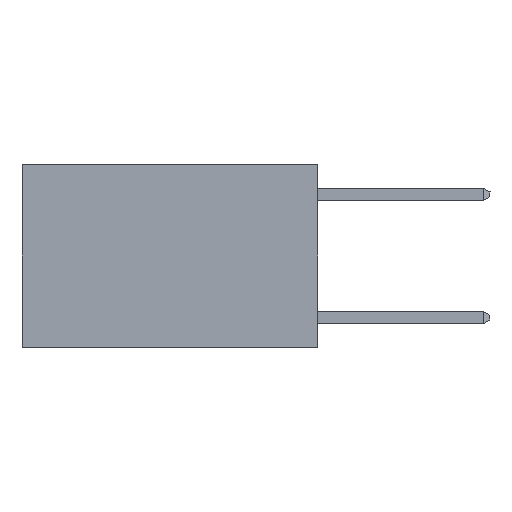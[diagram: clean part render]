
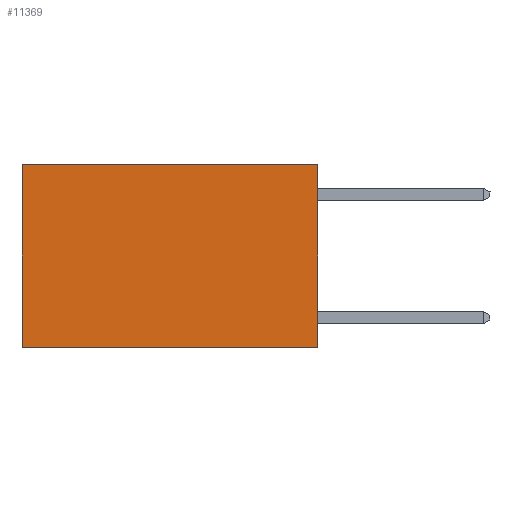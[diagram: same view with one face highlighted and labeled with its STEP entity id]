
A CAD part, left-side view. The second image highlights one B-rep face of the part: STEP entity #11369.
In plain terms, the highlighted planar face has unit normal (-1, 0, 0).
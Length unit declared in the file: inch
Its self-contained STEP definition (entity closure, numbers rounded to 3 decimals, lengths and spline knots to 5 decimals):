
#688 = CARTESIAN_POINT ( 'NONE',  ( 0.2625, 0., 0. ) ) ;
#1517 = PLANE ( 'NONE',  #5953 ) ;
#1941 = CARTESIAN_POINT ( 'NONE',  ( 0.2625, 0., 0. ) ) ;
#2280 = LINE ( 'NONE', #6878, #8079 ) ;
#2660 = DIRECTION ( 'NONE',  ( 0., 0., -1. ) ) ;
#2934 = EDGE_CURVE ( 'NONE', #7385, #6912, #9530, .T. ) ;
#2999 = ORIENTED_EDGE ( 'NONE', *, *, #4480, .F. ) ;
#3483 = ORIENTED_EDGE ( 'NONE', *, *, #5432, .F. ) ;
#3580 = VERTEX_POINT ( 'NONE', #11262 ) ;
#3749 = VECTOR ( 'NONE', #12425, 39.37008 ) ;
#4480 = EDGE_CURVE ( 'NONE', #7385, #3580, #8775, .T. ) ;
#5432 = EDGE_CURVE ( 'NONE', #3580, #12401, #2280, .T. ) ;
#5743 = DIRECTION ( 'NONE',  ( 0., 1., 0. ) ) ;
#5763 = ORIENTED_EDGE ( 'NONE', *, *, #2934, .T. ) ;
#5794 = EDGE_CURVE ( 'NONE', #6912, #12401, #9418, .T. ) ;
#5953 = AXIS2_PLACEMENT_3D ( 'NONE', #12424, #9156, #2660 ) ;
#6878 = CARTESIAN_POINT ( 'NONE',  ( 0.2625, 0., -0.37 ) ) ;
#6912 = VERTEX_POINT ( 'NONE', #8819 ) ;
#6995 = CARTESIAN_POINT ( 'NONE',  ( 0.2625, 0., 0. ) ) ;
#7261 = ORIENTED_EDGE ( 'NONE', *, *, #5794, .T. ) ;
#7385 = VERTEX_POINT ( 'NONE', #1941 ) ;
#7995 = CARTESIAN_POINT ( 'NONE',  ( 0.2625, 0.6, -0.37 ) ) ;
#8079 = VECTOR ( 'NONE', #5743, 39.37008 ) ;
#8102 = VECTOR ( 'NONE', #10570, 39.37008 ) ;
#8519 = CARTESIAN_POINT ( 'NONE',  ( 0.2625, 0.6, 0. ) ) ;
#8775 = LINE ( 'NONE', #688, #8102 ) ;
#8819 = CARTESIAN_POINT ( 'NONE',  ( 0.2625, 0.6, 0. ) ) ;
#9076 = VECTOR ( 'NONE', #10732, 39.37008 ) ;
#9156 = DIRECTION ( 'NONE',  ( 1., 0., 0. ) ) ;
#9418 = LINE ( 'NONE', #8519, #9076 ) ;
#9530 = LINE ( 'NONE', #6995, #3749 ) ;
#10570 = DIRECTION ( 'NONE',  ( 0., 0., -1. ) ) ;
#10732 = DIRECTION ( 'NONE',  ( 0., 0., -1. ) ) ;
#11262 = CARTESIAN_POINT ( 'NONE',  ( 0.2625, 0., -0.37 ) ) ;
#11369 = ADVANCED_FACE ( 'NONE', ( #14130 ), #1517, .F. ) ;
#12401 = VERTEX_POINT ( 'NONE', #7995 ) ;
#12424 = CARTESIAN_POINT ( 'NONE',  ( 0.2625, 0., 0. ) ) ;
#12425 = DIRECTION ( 'NONE',  ( 0., 1., 0. ) ) ;
#13920 = EDGE_LOOP ( 'NONE', ( #7261, #3483, #2999, #5763 ) ) ;
#14130 = FACE_OUTER_BOUND ( 'NONE', #13920, .T. ) ;
